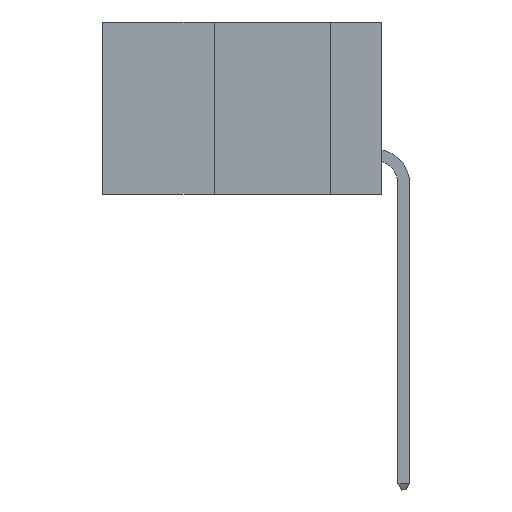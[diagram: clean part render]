
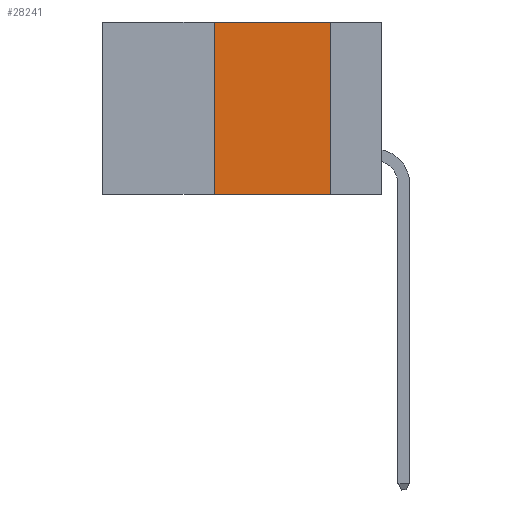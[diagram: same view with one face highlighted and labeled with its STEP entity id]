
A CAD part, left-side view. The second image highlights one B-rep face of the part: STEP entity #28241.
In plain terms, the highlighted planar face has unit normal (-1, 0, 0).
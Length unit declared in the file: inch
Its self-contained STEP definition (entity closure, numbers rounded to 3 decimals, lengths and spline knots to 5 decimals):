
#130 = PLANE ( 'NONE',  #9349 ) ;
#1555 = LINE ( 'NONE', #12139, #24928 ) ;
#2570 = DIRECTION ( 'NONE',  ( 0., 0., -1. ) ) ;
#2635 = ORIENTED_EDGE ( 'NONE', *, *, #6156, .T. ) ;
#3299 = LINE ( 'NONE', #5791, #27400 ) ;
#3900 = VERTEX_POINT ( 'NONE', #16338 ) ;
#5439 = CARTESIAN_POINT ( 'NONE',  ( 0., 0.36, 0. ) ) ;
#5791 = CARTESIAN_POINT ( 'NONE',  ( 0., 0.6, 0. ) ) ;
#6156 = EDGE_CURVE ( 'NONE', #3900, #6389, #26768, .T. ) ;
#6389 = VERTEX_POINT ( 'NONE', #30620 ) ;
#8181 = DIRECTION ( 'NONE',  ( 0., -1., 0. ) ) ;
#8435 = ORIENTED_EDGE ( 'NONE', *, *, #11570, .F. ) ;
#9349 = AXIS2_PLACEMENT_3D ( 'NONE', #14765, #12244, #24140 ) ;
#11570 = EDGE_CURVE ( 'NONE', #3900, #30995, #26829, .T. ) ;
#12113 = CARTESIAN_POINT ( 'NONE',  ( 0., 0.11, 0. ) ) ;
#12139 = CARTESIAN_POINT ( 'NONE',  ( 0., 0.11, 0. ) ) ;
#12244 = DIRECTION ( 'NONE',  ( 1., 0., 0. ) ) ;
#14061 = EDGE_CURVE ( 'NONE', #30995, #27706, #3299, .T. ) ;
#14694 = VECTOR ( 'NONE', #25640, 39.37008 ) ;
#14765 = CARTESIAN_POINT ( 'NONE',  ( 0., 0.6, 0. ) ) ;
#15114 = CARTESIAN_POINT ( 'NONE',  ( 0., 0.36, 0. ) ) ;
#15407 = ORIENTED_EDGE ( 'NONE', *, *, #18290, .F. ) ;
#16338 = CARTESIAN_POINT ( 'NONE',  ( 0., 0.36, -0.37 ) ) ;
#18290 = EDGE_CURVE ( 'NONE', #27706, #6389, #1555, .T. ) ;
#20707 = EDGE_LOOP ( 'NONE', ( #15407, #27160, #8435, #2635 ) ) ;
#21106 = DIRECTION ( 'NONE',  ( 0., 0., 1. ) ) ;
#23426 = VECTOR ( 'NONE', #21106, 39.37008 ) ;
#24140 = DIRECTION ( 'NONE',  ( 0., 0., -1. ) ) ;
#24928 = VECTOR ( 'NONE', #2570, 39.37008 ) ;
#25640 = DIRECTION ( 'NONE',  ( 0., -1., 0. ) ) ;
#26768 = LINE ( 'NONE', #27367, #14694 ) ;
#26829 = LINE ( 'NONE', #5439, #23426 ) ;
#27160 = ORIENTED_EDGE ( 'NONE', *, *, #14061, .F. ) ;
#27367 = CARTESIAN_POINT ( 'NONE',  ( 0., 0.6, -0.37 ) ) ;
#27369 = FACE_OUTER_BOUND ( 'NONE', #20707, .T. ) ;
#27400 = VECTOR ( 'NONE', #8181, 39.37008 ) ;
#27706 = VERTEX_POINT ( 'NONE', #12113 ) ;
#28241 = ADVANCED_FACE ( 'NONE', ( #27369 ), #130, .F. ) ;
#30620 = CARTESIAN_POINT ( 'NONE',  ( 0., 0.11, -0.37 ) ) ;
#30995 = VERTEX_POINT ( 'NONE', #15114 ) ;
